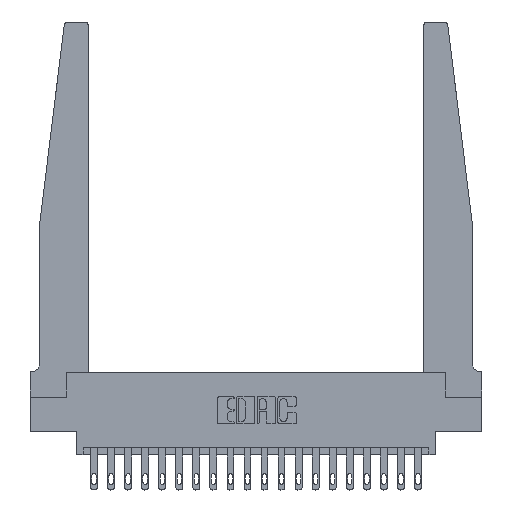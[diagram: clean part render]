
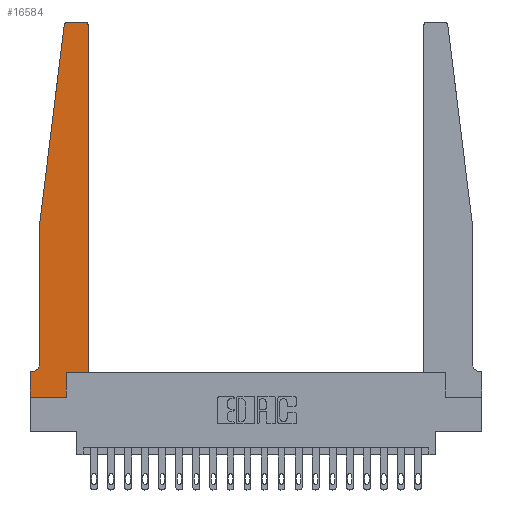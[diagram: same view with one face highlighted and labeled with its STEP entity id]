
A CAD part, top view. The second image highlights one B-rep face of the part: STEP entity #16584.
In plain terms, the highlighted planar face has unit normal (0, 0, 1).
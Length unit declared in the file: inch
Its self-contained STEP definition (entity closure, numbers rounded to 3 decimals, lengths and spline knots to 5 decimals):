
#71 = DIRECTION ( 'NONE',  ( 1., 0., 0. ) ) ;
#455 = DIRECTION ( 'NONE',  ( 0., 0., -1. ) ) ;
#626 = VERTEX_POINT ( 'NONE', #17669 ) ;
#1128 = CARTESIAN_POINT ( 'NONE',  ( 0., 0., 0.37 ) ) ;
#1161 = EDGE_CURVE ( 'NONE', #626, #4028, #16363, .T. ) ;
#1163 = CARTESIAN_POINT ( 'NONE',  ( 0.065, 1.25, 0.37 ) ) ;
#1407 = DIRECTION ( 'NONE',  ( 0., 1., 0. ) ) ;
#1589 = DIRECTION ( 'NONE',  ( 0., -1., 0. ) ) ;
#1675 = AXIS2_PLACEMENT_3D ( 'NONE', #4913, #6524, #7895 ) ;
#1787 = ORIENTED_EDGE ( 'NONE', *, *, #19532, .T. ) ;
#2127 = LINE ( 'NONE', #12287, #3696 ) ;
#2414 = ORIENTED_EDGE ( 'NONE', *, *, #11825, .T. ) ;
#2691 = VECTOR ( 'NONE', #15395, 39.37008 ) ;
#2835 = LINE ( 'NONE', #14364, #19718 ) ;
#3541 = CARTESIAN_POINT ( 'NONE',  ( 0.425, 0.18, 0.37 ) ) ;
#3650 = CARTESIAN_POINT ( 'NONE',  ( 0.2605, 0., 0.37 ) ) ;
#3696 = VECTOR ( 'NONE', #6900, 39.37008 ) ;
#4028 = VERTEX_POINT ( 'NONE', #13789 ) ;
#4032 = ORIENTED_EDGE ( 'NONE', *, *, #18918, .T. ) ;
#4042 = VERTEX_POINT ( 'NONE', #1163 ) ;
#4114 = CIRCLE ( 'NONE', #6215, 0.03 ) ;
#4119 = ORIENTED_EDGE ( 'NONE', *, *, #5452, .T. ) ;
#4605 = AXIS2_PLACEMENT_3D ( 'NONE', #6739, #18087, #71 ) ;
#4628 = CARTESIAN_POINT ( 'NONE',  ( 0.065, 0.2375, 0.37 ) ) ;
#4913 = CARTESIAN_POINT ( 'NONE',  ( 0., 0.1875, 0.37 ) ) ;
#5313 = DIRECTION ( 'NONE',  ( -1., 0., 0. ) ) ;
#5452 = EDGE_CURVE ( 'NONE', #13502, #18368, #5612, .T. ) ;
#5543 = ORIENTED_EDGE ( 'NONE', *, *, #9978, .T. ) ;
#5612 = CIRCLE ( 'NONE', #15958, 0.05 ) ;
#5647 = EDGE_CURVE ( 'NONE', #14746, #17352, #13915, .T. ) ;
#5918 = ORIENTED_EDGE ( 'NONE', *, *, #14985, .T. ) ;
#6215 = AXIS2_PLACEMENT_3D ( 'NONE', #10402, #8439, #14999 ) ;
#6322 = DIRECTION ( 'NONE',  ( 1., 0., 0. ) ) ;
#6443 = DIRECTION ( 'NONE',  ( 0., -1., 0. ) ) ;
#6524 = DIRECTION ( 'NONE',  ( 0., 0., 1. ) ) ;
#6656 = CIRCLE ( 'NONE', #4605, 0.03 ) ;
#6739 = CARTESIAN_POINT ( 'NONE',  ( 0.27653, 2.72, 0.37 ) ) ;
#6900 = DIRECTION ( 'NONE',  ( -0.122, -0.992, 0. ) ) ;
#7445 = DIRECTION ( 'NONE',  ( -1., 0., 0. ) ) ;
#7460 = VERTEX_POINT ( 'NONE', #3650 ) ;
#7804 = VECTOR ( 'NONE', #6443, 39.37008 ) ;
#7895 = DIRECTION ( 'NONE',  ( 1., 0., 0. ) ) ;
#8290 = ORIENTED_EDGE ( 'NONE', *, *, #19801, .T. ) ;
#8439 = DIRECTION ( 'NONE',  ( 0., 0., 1. ) ) ;
#8672 = CARTESIAN_POINT ( 'NONE',  ( 0.395, 2.75, 0.37 ) ) ;
#8829 = VERTEX_POINT ( 'NONE', #12550 ) ;
#8930 = EDGE_CURVE ( 'NONE', #7460, #17947, #2835, .T. ) ;
#9349 = VECTOR ( 'NONE', #1589, 39.37008 ) ;
#9477 = CARTESIAN_POINT ( 'NONE',  ( 0., 0., 0.37 ) ) ;
#9518 = FACE_OUTER_BOUND ( 'NONE', #11454, .T. ) ;
#9974 = CARTESIAN_POINT ( 'NONE',  ( 0.065, 1.25, 0.37 ) ) ;
#9978 = EDGE_CURVE ( 'NONE', #8829, #13140, #16158, .T. ) ;
#10402 = CARTESIAN_POINT ( 'NONE',  ( 0.395, 2.72, 0.37 ) ) ;
#10914 = VECTOR ( 'NONE', #6322, 39.37008 ) ;
#11257 = LINE ( 'NONE', #1128, #10914 ) ;
#11326 = CARTESIAN_POINT ( 'NONE',  ( 0.425, 2.72, 0.37 ) ) ;
#11359 = EDGE_CURVE ( 'NONE', #18368, #626, #16928, .T. ) ;
#11400 = LINE ( 'NONE', #9974, #7804 ) ;
#11454 = EDGE_LOOP ( 'NONE', ( #15203, #8290, #1787, #5918, #4119, #20210, #12872, #4032, #21206, #2414, #5543, #19183 ) ) ;
#11801 = CARTESIAN_POINT ( 'NONE',  ( 0.015, 0.2375, 0.37 ) ) ;
#11825 = EDGE_CURVE ( 'NONE', #17947, #8829, #20227, .T. ) ;
#12237 = EDGE_CURVE ( 'NONE', #13140, #14746, #4114, .T. ) ;
#12287 = CARTESIAN_POINT ( 'NONE',  ( 0.065, 1.25, 0.37 ) ) ;
#12358 = VECTOR ( 'NONE', #1407, 39.37008 ) ;
#12550 = CARTESIAN_POINT ( 'NONE',  ( 0.425, 0.18, 0.37 ) ) ;
#12574 = CARTESIAN_POINT ( 'NONE',  ( 0.015, 0.1875, 0.37 ) ) ;
#12698 = VECTOR ( 'NONE', #13779, 39.37008 ) ;
#12872 = ORIENTED_EDGE ( 'NONE', *, *, #1161, .T. ) ;
#13140 = VERTEX_POINT ( 'NONE', #11326 ) ;
#13502 = VERTEX_POINT ( 'NONE', #4628 ) ;
#13779 = DIRECTION ( 'NONE',  ( 1., 0., 0. ) ) ;
#13789 = CARTESIAN_POINT ( 'NONE',  ( 0., 0., 0.37 ) ) ;
#13915 = LINE ( 'NONE', #19216, #19785 ) ;
#14364 = CARTESIAN_POINT ( 'NONE',  ( 0.2605, 0.18, 0.37 ) ) ;
#14746 = VERTEX_POINT ( 'NONE', #8672 ) ;
#14985 = EDGE_CURVE ( 'NONE', #4042, #13502, #11400, .T. ) ;
#14990 = CARTESIAN_POINT ( 'NONE',  ( 0.24675, 2.72367, 0.37 ) ) ;
#14999 = DIRECTION ( 'NONE',  ( 1., 0., 0. ) ) ;
#15175 = CARTESIAN_POINT ( 'NONE',  ( 0.065, 0.1875, 0.37 ) ) ;
#15203 = ORIENTED_EDGE ( 'NONE', *, *, #5647, .T. ) ;
#15395 = DIRECTION ( 'NONE',  ( -1., 0., 0. ) ) ;
#15958 = AXIS2_PLACEMENT_3D ( 'NONE', #11801, #455, #5313 ) ;
#16080 = PLANE ( 'NONE',  #1675 ) ;
#16158 = LINE ( 'NONE', #17806, #12358 ) ;
#16363 = LINE ( 'NONE', #9477, #9349 ) ;
#16584 = ADVANCED_FACE ( 'NONE', ( #9518 ), #16080, .T. ) ;
#16928 = LINE ( 'NONE', #15175, #2691 ) ;
#17041 = VERTEX_POINT ( 'NONE', #14990 ) ;
#17352 = VERTEX_POINT ( 'NONE', #19032 ) ;
#17555 = CARTESIAN_POINT ( 'NONE',  ( 0.2605, 0.18, 0.37 ) ) ;
#17669 = CARTESIAN_POINT ( 'NONE',  ( 0., 0.1875, 0.37 ) ) ;
#17806 = CARTESIAN_POINT ( 'NONE',  ( 0.425, 0.18, 0.37 ) ) ;
#17947 = VERTEX_POINT ( 'NONE', #17555 ) ;
#18087 = DIRECTION ( 'NONE',  ( 0., 0., 1. ) ) ;
#18368 = VERTEX_POINT ( 'NONE', #12574 ) ;
#18918 = EDGE_CURVE ( 'NONE', #4028, #7460, #11257, .T. ) ;
#19032 = CARTESIAN_POINT ( 'NONE',  ( 0.27653, 2.75, 0.37 ) ) ;
#19183 = ORIENTED_EDGE ( 'NONE', *, *, #12237, .T. ) ;
#19216 = CARTESIAN_POINT ( 'NONE',  ( 0.25, 2.75, 0.37 ) ) ;
#19532 = EDGE_CURVE ( 'NONE', #17041, #4042, #2127, .T. ) ;
#19718 = VECTOR ( 'NONE', #20924, 39.37008 ) ;
#19785 = VECTOR ( 'NONE', #7445, 39.37008 ) ;
#19801 = EDGE_CURVE ( 'NONE', #17352, #17041, #6656, .T. ) ;
#20210 = ORIENTED_EDGE ( 'NONE', *, *, #11359, .T. ) ;
#20227 = LINE ( 'NONE', #3541, #12698 ) ;
#20924 = DIRECTION ( 'NONE',  ( 0., 1., 0. ) ) ;
#21206 = ORIENTED_EDGE ( 'NONE', *, *, #8930, .T. ) ;
